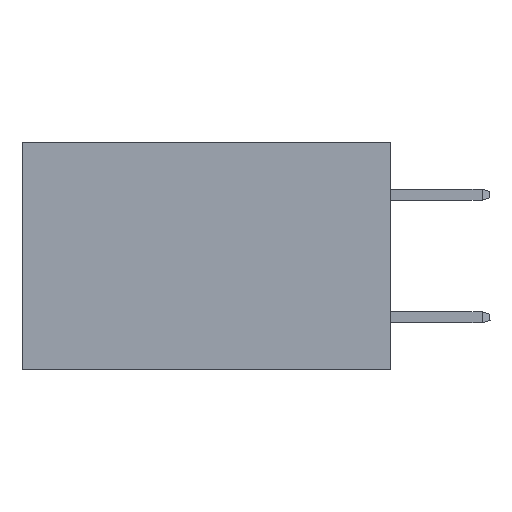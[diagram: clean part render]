
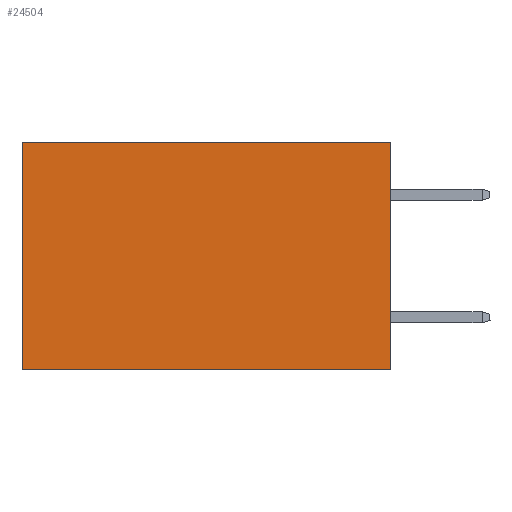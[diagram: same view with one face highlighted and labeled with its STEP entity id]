
A CAD part, left-side view. The second image highlights one B-rep face of the part: STEP entity #24504.
In plain terms, the highlighted planar face has unit normal (-1, 0, 0).
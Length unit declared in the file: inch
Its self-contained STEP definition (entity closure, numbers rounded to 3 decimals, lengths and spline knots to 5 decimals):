
#2921 = AXIS2_PLACEMENT_3D ( 'NONE', #8234, #24420, #14840 ) ;
#4042 = VERTEX_POINT ( 'NONE', #5591 ) ;
#4897 = CARTESIAN_POINT ( 'NONE',  ( 0.2875, 0., -0.37 ) ) ;
#5591 = CARTESIAN_POINT ( 'NONE',  ( 0.2875, 0., -0.37 ) ) ;
#5681 = ORIENTED_EDGE ( 'NONE', *, *, #41450, .T. ) ;
#8069 = VECTOR ( 'NONE', #29002, 39.37008 ) ;
#8234 = CARTESIAN_POINT ( 'NONE',  ( 0.2875, 0., 0. ) ) ;
#11736 = VERTEX_POINT ( 'NONE', #37559 ) ;
#14565 = PLANE ( 'NONE',  #2921 ) ;
#14840 = DIRECTION ( 'NONE',  ( 0., 0., -1. ) ) ;
#15788 = VERTEX_POINT ( 'NONE', #17373 ) ;
#16886 = VECTOR ( 'NONE', #42494, 39.37008 ) ;
#17373 = CARTESIAN_POINT ( 'NONE',  ( 0.2875, 0.6, -0.37 ) ) ;
#17934 = EDGE_CURVE ( 'NONE', #4042, #15788, #35180, .T. ) ;
#18265 = VERTEX_POINT ( 'NONE', #38731 ) ;
#18755 = CARTESIAN_POINT ( 'NONE',  ( 0.2875, 0.6, 0. ) ) ;
#21860 = EDGE_LOOP ( 'NONE', ( #5681, #26819, #39448, #22115 ) ) ;
#22115 = ORIENTED_EDGE ( 'NONE', *, *, #39122, .T. ) ;
#23905 = VECTOR ( 'NONE', #34461, 39.37008 ) ;
#24420 = DIRECTION ( 'NONE',  ( 1., 0., 0. ) ) ;
#24504 = ADVANCED_FACE ( 'NONE', ( #31076 ), #14565, .F. ) ;
#25170 = DIRECTION ( 'NONE',  ( 0., 0., -1. ) ) ;
#25594 = LINE ( 'NONE', #29734, #16886 ) ;
#26819 = ORIENTED_EDGE ( 'NONE', *, *, #17934, .F. ) ;
#28451 = EDGE_CURVE ( 'NONE', #18265, #4042, #25594, .T. ) ;
#29002 = DIRECTION ( 'NONE',  ( 0., 1., 0. ) ) ;
#29734 = CARTESIAN_POINT ( 'NONE',  ( 0.2875, 0., 0. ) ) ;
#30949 = LINE ( 'NONE', #18755, #38610 ) ;
#31076 = FACE_OUTER_BOUND ( 'NONE', #21860, .T. ) ;
#34461 = DIRECTION ( 'NONE',  ( 0., 1., 0. ) ) ;
#35180 = LINE ( 'NONE', #4897, #23905 ) ;
#37559 = CARTESIAN_POINT ( 'NONE',  ( 0.2875, 0.6, 0. ) ) ;
#38610 = VECTOR ( 'NONE', #25170, 39.37008 ) ;
#38731 = CARTESIAN_POINT ( 'NONE',  ( 0.2875, 0., 0. ) ) ;
#39122 = EDGE_CURVE ( 'NONE', #18265, #11736, #41895, .T. ) ;
#39448 = ORIENTED_EDGE ( 'NONE', *, *, #28451, .F. ) ;
#41450 = EDGE_CURVE ( 'NONE', #11736, #15788, #30949, .T. ) ;
#41895 = LINE ( 'NONE', #42461, #8069 ) ;
#42461 = CARTESIAN_POINT ( 'NONE',  ( 0.2875, 0., 0. ) ) ;
#42494 = DIRECTION ( 'NONE',  ( 0., 0., -1. ) ) ;
